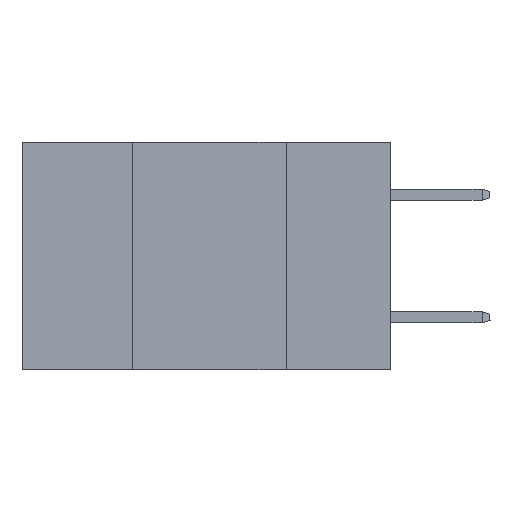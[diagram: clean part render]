
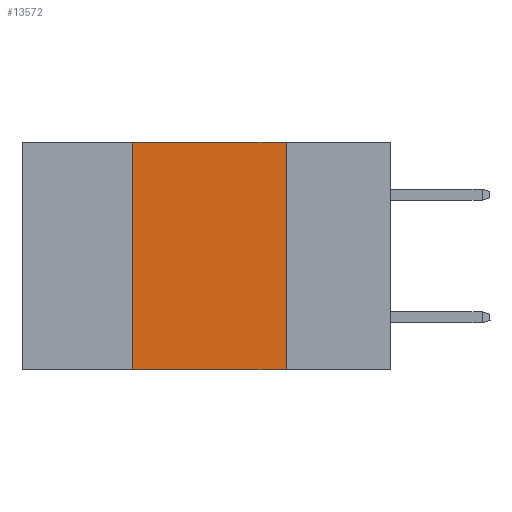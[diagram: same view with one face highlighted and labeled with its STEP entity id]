
A CAD part, left-side view. The second image highlights one B-rep face of the part: STEP entity #13572.
In plain terms, the highlighted planar face has unit normal (-1, 0, 0).
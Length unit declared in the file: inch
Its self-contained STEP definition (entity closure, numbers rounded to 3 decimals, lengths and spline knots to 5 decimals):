
#517 = EDGE_CURVE ( 'NONE', #17425, #11464, #1507, .T. ) ;
#1278 = DIRECTION ( 'NONE',  ( 0., -1., 0. ) ) ;
#1507 = LINE ( 'NONE', #4862, #14681 ) ;
#1932 = CARTESIAN_POINT ( 'NONE',  ( 0., 0.42, 0. ) ) ;
#2055 = VECTOR ( 'NONE', #12940, 39.37008 ) ;
#2344 = CARTESIAN_POINT ( 'NONE',  ( 0., 0.6, 0. ) ) ;
#2526 = VERTEX_POINT ( 'NONE', #21072 ) ;
#2636 = CARTESIAN_POINT ( 'NONE',  ( 0., 0.6, 0. ) ) ;
#2935 = AXIS2_PLACEMENT_3D ( 'NONE', #2344, #5868, #17793 ) ;
#3704 = DIRECTION ( 'NONE',  ( 0., 0., 1. ) ) ;
#4261 = FACE_OUTER_BOUND ( 'NONE', #4969, .T. ) ;
#4862 = CARTESIAN_POINT ( 'NONE',  ( 0., 0.6, -0.37 ) ) ;
#4969 = EDGE_LOOP ( 'NONE', ( #6446, #14206, #10263, #21687 ) ) ;
#5868 = DIRECTION ( 'NONE',  ( 1., 0., 0. ) ) ;
#6446 = ORIENTED_EDGE ( 'NONE', *, *, #12114, .F. ) ;
#6677 = LINE ( 'NONE', #2636, #2055 ) ;
#7502 = EDGE_CURVE ( 'NONE', #17425, #11879, #21468, .T. ) ;
#9293 = CARTESIAN_POINT ( 'NONE',  ( 0., 0.42, -0.37 ) ) ;
#10263 = ORIENTED_EDGE ( 'NONE', *, *, #7502, .F. ) ;
#11464 = VERTEX_POINT ( 'NONE', #20055 ) ;
#11879 = VERTEX_POINT ( 'NONE', #19542 ) ;
#12114 = EDGE_CURVE ( 'NONE', #2526, #11464, #21302, .T. ) ;
#12419 = VECTOR ( 'NONE', #21698, 39.37008 ) ;
#12587 = EDGE_CURVE ( 'NONE', #11879, #2526, #6677, .T. ) ;
#12940 = DIRECTION ( 'NONE',  ( 0., -1., 0. ) ) ;
#13572 = ADVANCED_FACE ( 'NONE', ( #4261 ), #16113, .F. ) ;
#14206 = ORIENTED_EDGE ( 'NONE', *, *, #12587, .F. ) ;
#14681 = VECTOR ( 'NONE', #1278, 39.37008 ) ;
#16113 = PLANE ( 'NONE',  #2935 ) ;
#17124 = VECTOR ( 'NONE', #3704, 39.37008 ) ;
#17425 = VERTEX_POINT ( 'NONE', #9293 ) ;
#17793 = DIRECTION ( 'NONE',  ( 0., 0., -1. ) ) ;
#19542 = CARTESIAN_POINT ( 'NONE',  ( 0., 0.42, 0. ) ) ;
#20055 = CARTESIAN_POINT ( 'NONE',  ( 0., 0.17, -0.37 ) ) ;
#20097 = CARTESIAN_POINT ( 'NONE',  ( 0., 0.17, 0. ) ) ;
#21072 = CARTESIAN_POINT ( 'NONE',  ( 0., 0.17, 0. ) ) ;
#21302 = LINE ( 'NONE', #20097, #12419 ) ;
#21468 = LINE ( 'NONE', #1932, #17124 ) ;
#21687 = ORIENTED_EDGE ( 'NONE', *, *, #517, .T. ) ;
#21698 = DIRECTION ( 'NONE',  ( 0., 0., -1. ) ) ;
